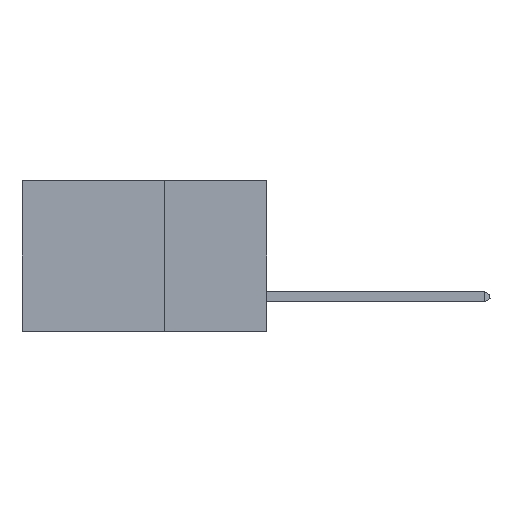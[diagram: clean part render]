
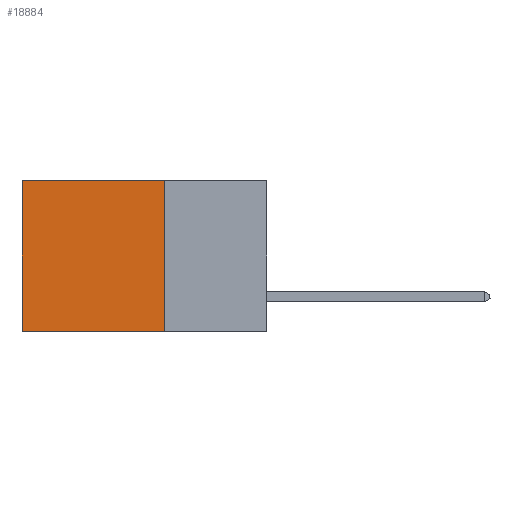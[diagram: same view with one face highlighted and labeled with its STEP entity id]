
A CAD part, left-side view. The second image highlights one B-rep face of the part: STEP entity #18884.
In plain terms, the highlighted planar face has unit normal (-1, 0, 0).
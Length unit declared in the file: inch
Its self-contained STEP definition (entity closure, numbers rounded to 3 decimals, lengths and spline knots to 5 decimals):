
#50 = VERTEX_POINT ( 'NONE', #380 ) ;
#380 = CARTESIAN_POINT ( 'NONE',  ( 0.2875, 0.6, -0.37 ) ) ;
#529 = CARTESIAN_POINT ( 'NONE',  ( 0.2875, 0.6, 0. ) ) ;
#1712 = DIRECTION ( 'NONE',  ( 1., 0., 0. ) ) ;
#1916 = CARTESIAN_POINT ( 'NONE',  ( 0.2875, 0.25, 0. ) ) ;
#2111 = VECTOR ( 'NONE', #24997, 39.37008 ) ;
#2748 = DIRECTION ( 'NONE',  ( 0., 1., 0. ) ) ;
#3524 = ORIENTED_EDGE ( 'NONE', *, *, #19157, .T. ) ;
#3741 = PLANE ( 'NONE',  #10476 ) ;
#4054 = LINE ( 'NONE', #25726, #4367 ) ;
#4367 = VECTOR ( 'NONE', #2748, 39.37008 ) ;
#4604 = ORIENTED_EDGE ( 'NONE', *, *, #22533, .F. ) ;
#7142 = VERTEX_POINT ( 'NONE', #16706 ) ;
#8338 = FACE_OUTER_BOUND ( 'NONE', #10301, .T. ) ;
#8473 = CARTESIAN_POINT ( 'NONE',  ( 0.2875, 0.25, 0. ) ) ;
#8508 = VERTEX_POINT ( 'NONE', #15341 ) ;
#9391 = LINE ( 'NONE', #529, #11651 ) ;
#10301 = EDGE_LOOP ( 'NONE', ( #24626, #11674, #4604, #3524 ) ) ;
#10476 = AXIS2_PLACEMENT_3D ( 'NONE', #12140, #1712, #18949 ) ;
#11420 = DIRECTION ( 'NONE',  ( 0., 0., -1. ) ) ;
#11651 = VECTOR ( 'NONE', #11420, 39.37008 ) ;
#11674 = ORIENTED_EDGE ( 'NONE', *, *, #25920, .F. ) ;
#12140 = CARTESIAN_POINT ( 'NONE',  ( 0.2875, 0.25, 0. ) ) ;
#13767 = DIRECTION ( 'NONE',  ( 0., 1., 0. ) ) ;
#14043 = LINE ( 'NONE', #24307, #19976 ) ;
#15341 = CARTESIAN_POINT ( 'NONE',  ( 0.2875, 0.25, -0.37 ) ) ;
#15460 = VERTEX_POINT ( 'NONE', #8473 ) ;
#16706 = CARTESIAN_POINT ( 'NONE',  ( 0.2875, 0.6, 0. ) ) ;
#17649 = EDGE_CURVE ( 'NONE', #7142, #50, #9391, .T. ) ;
#18884 = ADVANCED_FACE ( 'NONE', ( #8338 ), #3741, .F. ) ;
#18949 = DIRECTION ( 'NONE',  ( 0., 0., -1. ) ) ;
#19157 = EDGE_CURVE ( 'NONE', #15460, #7142, #4054, .T. ) ;
#19976 = VECTOR ( 'NONE', #13767, 39.37008 ) ;
#22533 = EDGE_CURVE ( 'NONE', #15460, #8508, #24497, .T. ) ;
#24307 = CARTESIAN_POINT ( 'NONE',  ( 0.2875, 0.25, -0.37 ) ) ;
#24497 = LINE ( 'NONE', #1916, #2111 ) ;
#24626 = ORIENTED_EDGE ( 'NONE', *, *, #17649, .T. ) ;
#24997 = DIRECTION ( 'NONE',  ( 0., 0., -1. ) ) ;
#25726 = CARTESIAN_POINT ( 'NONE',  ( 0.2875, 0.25, 0. ) ) ;
#25920 = EDGE_CURVE ( 'NONE', #8508, #50, #14043, .T. ) ;
